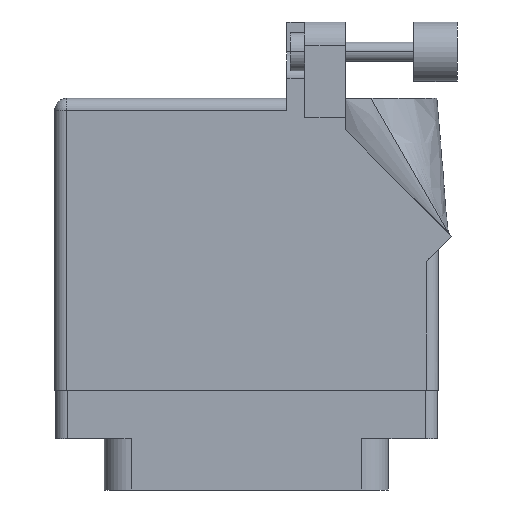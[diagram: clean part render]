
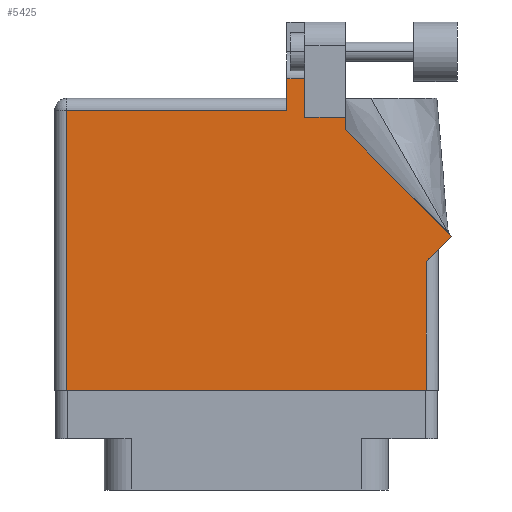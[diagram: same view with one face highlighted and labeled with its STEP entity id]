
A CAD part, front view. The second image highlights one B-rep face of the part: STEP entity #5425.
In plain terms, the highlighted face is planar.
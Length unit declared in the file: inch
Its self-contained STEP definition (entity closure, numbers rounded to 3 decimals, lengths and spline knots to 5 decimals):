
#878 = VECTOR ( 'NONE', #31843, 39.37008 ) ;
#960 = CARTESIAN_POINT ( 'NONE',  ( 1.07571, 0.70771, 0.455 ) ) ;
#1365 = ORIENTED_EDGE ( 'NONE', *, *, #14441, .T. ) ;
#1895 = DIRECTION ( 'NONE',  ( 0., 1., 0. ) ) ;
#2259 = VERTEX_POINT ( 'NONE', #24513 ) ;
#2296 = CARTESIAN_POINT ( 'NONE',  ( -1.005, 1.43, 0.455 ) ) ;
#2396 = DIRECTION ( 'NONE',  ( 0., 1., 0. ) ) ;
#2570 = DIRECTION ( 'NONE',  ( 0., 1., 0. ) ) ;
#2948 = CARTESIAN_POINT ( 'NONE',  ( 0.943, 0.575, 0.455 ) ) ;
#3212 = DIRECTION ( 'NONE',  ( -1., 0., 0. ) ) ;
#3247 = VERTEX_POINT ( 'NONE', #20180 ) ;
#3998 = LINE ( 'NONE', #36084, #16307 ) ;
#4272 = VECTOR ( 'NONE', #10156, 39.37008 ) ;
#4945 = LINE ( 'NONE', #25857, #15933 ) ;
#5184 = VECTOR ( 'NONE', #1895, 39.37008 ) ;
#5425 = ADVANCED_FACE ( 'NONE', ( #34638 ), #13616, .F. ) ;
#5968 = VECTOR ( 'NONE', #2396, 39.37008 ) ;
#6057 = ORIENTED_EDGE ( 'NONE', *, *, #6183, .T. ) ;
#6183 = EDGE_CURVE ( 'NONE', #22490, #3247, #18365, .T. ) ;
#6567 = CARTESIAN_POINT ( 'NONE',  ( 0.306, 1.33, 0.455 ) ) ;
#6860 = LINE ( 'NONE', #30863, #5968 ) ;
#7574 = CARTESIAN_POINT ( 'NONE',  ( 1.07571, 0.70771, 0.455 ) ) ;
#7746 = VERTEX_POINT ( 'NONE', #17343 ) ;
#8041 = VECTOR ( 'NONE', #9842, 39.37008 ) ;
#8112 = EDGE_CURVE ( 'NONE', #7746, #18243, #16081, .T. ) ;
#8132 = EDGE_CURVE ( 'NONE', #24095, #35996, #33620, .T. ) ;
#8638 = CARTESIAN_POINT ( 'NONE',  ( -1.005, 1.368, 0.455 ) ) ;
#9009 = LINE ( 'NONE', #8638, #16467 ) ;
#9842 = DIRECTION ( 'NONE',  ( 0., -1., 0. ) ) ;
#10156 = DIRECTION ( 'NONE',  ( -0.707, 0.707, 0. ) ) ;
#10498 = CARTESIAN_POINT ( 'NONE',  ( 0.943, 0.637, 0.455 ) ) ;
#11148 = ORIENTED_EDGE ( 'NONE', *, *, #13298, .T. ) ;
#12418 = EDGE_CURVE ( 'NONE', #32109, #28762, #31309, .T. ) ;
#13298 = EDGE_CURVE ( 'NONE', #18243, #2259, #3998, .T. ) ;
#13616 = PLANE ( 'NONE',  #17373 ) ;
#13950 = ORIENTED_EDGE ( 'NONE', *, *, #12418, .T. ) ;
#14441 = EDGE_CURVE ( 'NONE', #23595, #22490, #14660, .T. ) ;
#14592 = ORIENTED_EDGE ( 'NONE', *, *, #8112, .T. ) ;
#14660 = LINE ( 'NONE', #29419, #33080 ) ;
#14884 = LINE ( 'NONE', #10498, #5184 ) ;
#14931 = LINE ( 'NONE', #17543, #878 ) ;
#15769 = EDGE_LOOP ( 'NONE', ( #11148, #32691, #13950, #25942, #31676, #21602, #15930, #1365, #6057, #34172, #14592 ) ) ;
#15930 = ORIENTED_EDGE ( 'NONE', *, *, #34887, .T. ) ;
#15933 = VECTOR ( 'NONE', #20346, 39.37008 ) ;
#16081 = LINE ( 'NONE', #17124, #25297 ) ;
#16307 = VECTOR ( 'NONE', #2570, 39.37008 ) ;
#16362 = EDGE_CURVE ( 'NONE', #2259, #32109, #14931, .T. ) ;
#16467 = VECTOR ( 'NONE', #3212, 39.37008 ) ;
#17124 = CARTESIAN_POINT ( 'NONE',  ( 0.519, 1.33, 0.455 ) ) ;
#17343 = CARTESIAN_POINT ( 'NONE',  ( 0.519, 1.33, 0.455 ) ) ;
#17373 = AXIS2_PLACEMENT_3D ( 'NONE', #2296, #22292, #27685 ) ;
#17543 = CARTESIAN_POINT ( 'NONE',  ( 0.63677, 1.5315, 0.455 ) ) ;
#18238 = VECTOR ( 'NONE', #22366, 39.37008 ) ;
#18243 = VERTEX_POINT ( 'NONE', #6567 ) ;
#18365 = LINE ( 'NONE', #7574, #4272 ) ;
#19524 = EDGE_CURVE ( 'NONE', #28762, #24095, #9009, .T. ) ;
#19685 = DIRECTION ( 'NONE',  ( -1., 0., 0. ) ) ;
#19929 = VERTEX_POINT ( 'NONE', #33260 ) ;
#20047 = CARTESIAN_POINT ( 'NONE',  ( 0.212, 1.5315, 0.455 ) ) ;
#20180 = CARTESIAN_POINT ( 'NONE',  ( 0.519, 1.26442, 0.455 ) ) ;
#20346 = DIRECTION ( 'NONE',  ( 1., 0., 0. ) ) ;
#21268 = CARTESIAN_POINT ( 'NONE',  ( 0.212, 1.43, 0.455 ) ) ;
#21478 = CARTESIAN_POINT ( 'NONE',  ( -0.943, -0.1, 0.455 ) ) ;
#21602 = ORIENTED_EDGE ( 'NONE', *, *, #24235, .T. ) ;
#22292 = DIRECTION ( 'NONE',  ( 0., 0., -1. ) ) ;
#22366 = DIRECTION ( 'NONE',  ( 0., -1., 0. ) ) ;
#22490 = VERTEX_POINT ( 'NONE', #960 ) ;
#23595 = VERTEX_POINT ( 'NONE', #2948 ) ;
#24095 = VERTEX_POINT ( 'NONE', #25247 ) ;
#24235 = EDGE_CURVE ( 'NONE', #35996, #19929, #4945, .T. ) ;
#24513 = CARTESIAN_POINT ( 'NONE',  ( 0.306, 1.5315, 0.455 ) ) ;
#25247 = CARTESIAN_POINT ( 'NONE',  ( -0.943, 1.368, 0.455 ) ) ;
#25297 = VECTOR ( 'NONE', #19685, 39.37008 ) ;
#25857 = CARTESIAN_POINT ( 'NONE',  ( -1.005, -0.1, 0.455 ) ) ;
#25942 = ORIENTED_EDGE ( 'NONE', *, *, #19524, .T. ) ;
#26822 = CARTESIAN_POINT ( 'NONE',  ( 0.212, 1.368, 0.455 ) ) ;
#27685 = DIRECTION ( 'NONE',  ( -1., 0., 0. ) ) ;
#28762 = VERTEX_POINT ( 'NONE', #26822 ) ;
#29069 = EDGE_CURVE ( 'NONE', #3247, #7746, #6860, .T. ) ;
#29419 = CARTESIAN_POINT ( 'NONE',  ( 1.005, 0.637, 0.455 ) ) ;
#30863 = CARTESIAN_POINT ( 'NONE',  ( 0.519, 1.26442, 0.455 ) ) ;
#31309 = LINE ( 'NONE', #21268, #8041 ) ;
#31676 = ORIENTED_EDGE ( 'NONE', *, *, #8132, .T. ) ;
#31843 = DIRECTION ( 'NONE',  ( -1., 0., 0. ) ) ;
#32109 = VERTEX_POINT ( 'NONE', #20047 ) ;
#32256 = DIRECTION ( 'NONE',  ( 0.707, 0.707, 0. ) ) ;
#32691 = ORIENTED_EDGE ( 'NONE', *, *, #16362, .T. ) ;
#33080 = VECTOR ( 'NONE', #32256, 39.37008 ) ;
#33260 = CARTESIAN_POINT ( 'NONE',  ( 0.943, -0.1, 0.455 ) ) ;
#33620 = LINE ( 'NONE', #34034, #18238 ) ;
#34034 = CARTESIAN_POINT ( 'NONE',  ( -0.943, -0.1, 0.455 ) ) ;
#34172 = ORIENTED_EDGE ( 'NONE', *, *, #29069, .T. ) ;
#34638 = FACE_OUTER_BOUND ( 'NONE', #15769, .T. ) ;
#34887 = EDGE_CURVE ( 'NONE', #19929, #23595, #14884, .T. ) ;
#35996 = VERTEX_POINT ( 'NONE', #21478 ) ;
#36084 = CARTESIAN_POINT ( 'NONE',  ( 0.306, 1.33, 0.455 ) ) ;
